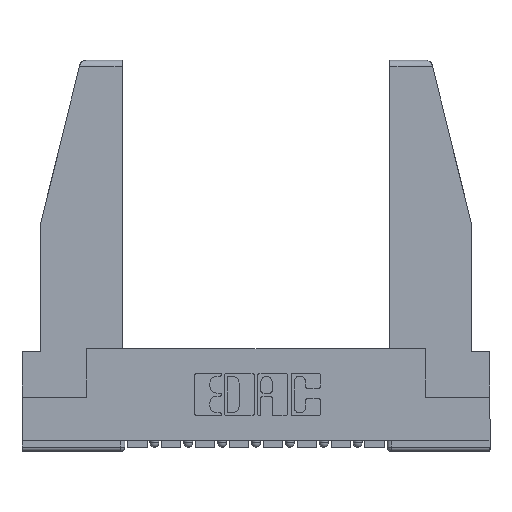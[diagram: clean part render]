
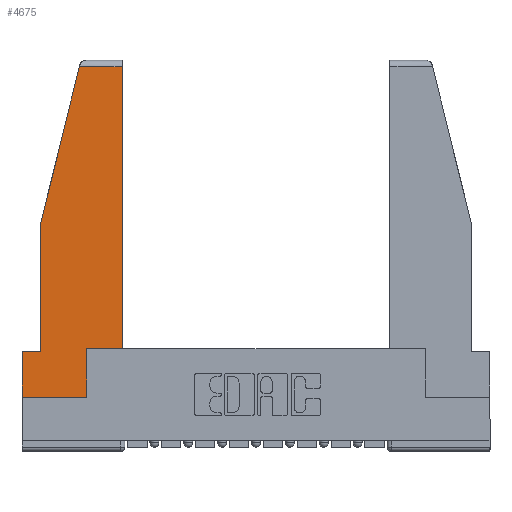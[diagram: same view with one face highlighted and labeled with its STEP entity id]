
A CAD part, top view. The second image highlights one B-rep face of the part: STEP entity #4675.
In plain terms, the highlighted planar face has unit normal (0, 0, 1).
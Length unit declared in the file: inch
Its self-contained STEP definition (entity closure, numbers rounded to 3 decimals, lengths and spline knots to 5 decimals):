
#152 = EDGE_CURVE ( 'NONE', #9076, #4134, #11312, .T. ) ;
#359 = ORIENTED_EDGE ( 'NONE', *, *, #456, .T. ) ;
#453 = AXIS2_PLACEMENT_3D ( 'NONE', #896, #8564, #4127 ) ;
#456 = EDGE_CURVE ( 'NONE', #6550, #7231, #9187, .T. ) ;
#460 = CARTESIAN_POINT ( 'NONE',  ( 0., 0., 0. ) ) ;
#512 = DIRECTION ( 'NONE',  ( 1., 0., 0. ) ) ;
#665 = CARTESIAN_POINT ( 'NONE',  ( 0.2636, 1.52, 0. ) ) ;
#668 = VERTEX_POINT ( 'NONE', #460 ) ;
#896 = CARTESIAN_POINT ( 'NONE',  ( 0., 0., 0. ) ) ;
#1556 = DIRECTION ( 'NONE',  ( 0., -1., 0. ) ) ;
#1569 = LINE ( 'NONE', #6563, #9936 ) ;
#1926 = LINE ( 'NONE', #12014, #13473 ) ;
#1936 = CARTESIAN_POINT ( 'NONE',  ( 0.086, 0.21, 0. ) ) ;
#1951 = EDGE_CURVE ( 'NONE', #12586, #9076, #12677, .T. ) ;
#2313 = VECTOR ( 'NONE', #512, 39.37008 ) ;
#2845 = ORIENTED_EDGE ( 'NONE', *, *, #6524, .T. ) ;
#2875 = DIRECTION ( 'NONE',  ( -1., 0., 0. ) ) ;
#3292 = DIRECTION ( 'NONE',  ( 0., 1., 0. ) ) ;
#3620 = EDGE_CURVE ( 'NONE', #4134, #4787, #1569, .T. ) ;
#3980 = CARTESIAN_POINT ( 'NONE',  ( 0., 0.21, 0. ) ) ;
#4039 = EDGE_CURVE ( 'NONE', #4787, #668, #7828, .T. ) ;
#4127 = DIRECTION ( 'NONE',  ( 1., 0., 0. ) ) ;
#4134 = VERTEX_POINT ( 'NONE', #1936 ) ;
#4437 = ORIENTED_EDGE ( 'NONE', *, *, #14429, .T. ) ;
#4653 = CARTESIAN_POINT ( 'NONE',  ( 0.461, 1.52, 0. ) ) ;
#4675 = ADVANCED_FACE ( 'NONE', ( #11330 ), #14122, .T. ) ;
#4787 = VERTEX_POINT ( 'NONE', #7719 ) ;
#4924 = CARTESIAN_POINT ( 'NONE',  ( 0., 0., 0. ) ) ;
#5203 = VECTOR ( 'NONE', #5571, 39.37008 ) ;
#5449 = VERTEX_POINT ( 'NONE', #4653 ) ;
#5535 = CARTESIAN_POINT ( 'NONE',  ( 0.297, 0., 0. ) ) ;
#5571 = DIRECTION ( 'NONE',  ( 0., -1., 0. ) ) ;
#6178 = EDGE_CURVE ( 'NONE', #668, #6550, #11208, .T. ) ;
#6223 = VECTOR ( 'NONE', #12157, 39.37008 ) ;
#6524 = EDGE_CURVE ( 'NONE', #13177, #5449, #12066, .T. ) ;
#6550 = VERTEX_POINT ( 'NONE', #5535 ) ;
#6563 = CARTESIAN_POINT ( 'NONE',  ( 0., 0.21, 0. ) ) ;
#6711 = VECTOR ( 'NONE', #8814, 39.37008 ) ;
#6908 = EDGE_LOOP ( 'NONE', ( #2845, #4437, #13708, #7972, #13214, #11360, #10024, #359, #11344 ) ) ;
#7231 = VERTEX_POINT ( 'NONE', #13606 ) ;
#7719 = CARTESIAN_POINT ( 'NONE',  ( 0., 0.21, 0. ) ) ;
#7828 = LINE ( 'NONE', #3980, #8369 ) ;
#7972 = ORIENTED_EDGE ( 'NONE', *, *, #152, .T. ) ;
#8366 = VECTOR ( 'NONE', #11705, 39.37008 ) ;
#8369 = VECTOR ( 'NONE', #1556, 39.37008 ) ;
#8478 = CARTESIAN_POINT ( 'NONE',  ( 0.461, 0.223, 0. ) ) ;
#8564 = DIRECTION ( 'NONE',  ( 0., 0., 1. ) ) ;
#8814 = DIRECTION ( 'NONE',  ( -0.239, -0.971, 0. ) ) ;
#8847 = CARTESIAN_POINT ( 'NONE',  ( 0.461, 0.223, 0. ) ) ;
#9076 = VERTEX_POINT ( 'NONE', #9896 ) ;
#9187 = LINE ( 'NONE', #9788, #6223 ) ;
#9788 = CARTESIAN_POINT ( 'NONE',  ( 0.297, 0., 0. ) ) ;
#9896 = CARTESIAN_POINT ( 'NONE',  ( 0.086, 0.8, 0. ) ) ;
#9936 = VECTOR ( 'NONE', #2875, 39.37008 ) ;
#9950 = DIRECTION ( 'NONE',  ( 1., 0., 0. ) ) ;
#10024 = ORIENTED_EDGE ( 'NONE', *, *, #6178, .T. ) ;
#10454 = LINE ( 'NONE', #13921, #8366 ) ;
#10651 = VECTOR ( 'NONE', #3292, 39.37008 ) ;
#11020 = CARTESIAN_POINT ( 'NONE',  ( 0.086, 0.8, 0. ) ) ;
#11208 = LINE ( 'NONE', #4924, #2313 ) ;
#11312 = LINE ( 'NONE', #11020, #5203 ) ;
#11330 = FACE_OUTER_BOUND ( 'NONE', #6908, .T. ) ;
#11344 = ORIENTED_EDGE ( 'NONE', *, *, #13923, .T. ) ;
#11360 = ORIENTED_EDGE ( 'NONE', *, *, #4039, .T. ) ;
#11705 = DIRECTION ( 'NONE',  ( -1., 0., 0. ) ) ;
#12014 = CARTESIAN_POINT ( 'NONE',  ( 0.297, 0.223, 0. ) ) ;
#12066 = LINE ( 'NONE', #8847, #10651 ) ;
#12157 = DIRECTION ( 'NONE',  ( 0., 1., 0. ) ) ;
#12586 = VERTEX_POINT ( 'NONE', #665 ) ;
#12677 = LINE ( 'NONE', #13273, #6711 ) ;
#13177 = VERTEX_POINT ( 'NONE', #8478 ) ;
#13214 = ORIENTED_EDGE ( 'NONE', *, *, #3620, .T. ) ;
#13273 = CARTESIAN_POINT ( 'NONE',  ( 0.271, 1.55, 0. ) ) ;
#13473 = VECTOR ( 'NONE', #9950, 39.37008 ) ;
#13606 = CARTESIAN_POINT ( 'NONE',  ( 0.297, 0.223, 0. ) ) ;
#13708 = ORIENTED_EDGE ( 'NONE', *, *, #1951, .T. ) ;
#13921 = CARTESIAN_POINT ( 'NONE',  ( 0., 1.52, 0. ) ) ;
#13923 = EDGE_CURVE ( 'NONE', #7231, #13177, #1926, .T. ) ;
#14122 = PLANE ( 'NONE',  #453 ) ;
#14429 = EDGE_CURVE ( 'NONE', #5449, #12586, #10454, .T. ) ;
